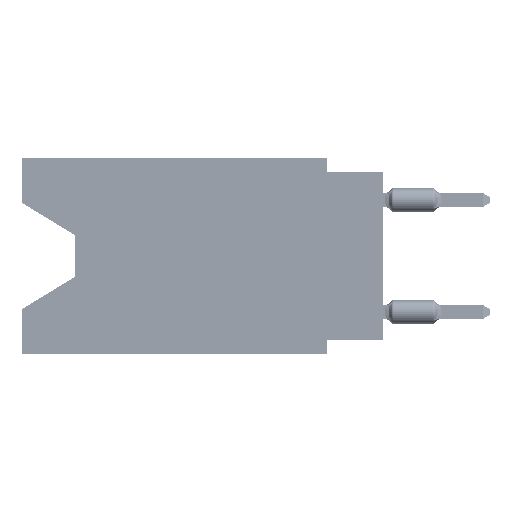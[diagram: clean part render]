
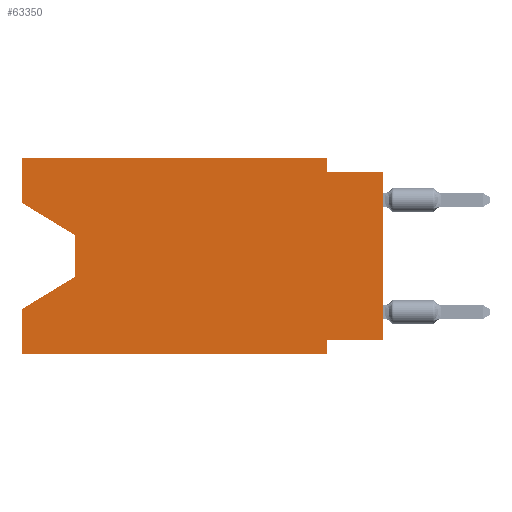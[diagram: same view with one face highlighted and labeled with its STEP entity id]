
A CAD part, left-side view. The second image highlights one B-rep face of the part: STEP entity #63350.
In plain terms, the highlighted planar face has unit normal (-1, 0, 0).
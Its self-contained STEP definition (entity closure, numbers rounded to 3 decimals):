
#516 = CARTESIAN_POINT ( 'NONE',  ( 0., 16.383, -8.89 ) ) ;
#523 = VERTEX_POINT ( 'NONE', #42212 ) ;
#1295 = ORIENTED_EDGE ( 'NONE', *, *, #9275, .T. ) ;
#1318 = CARTESIAN_POINT ( 'NONE',  ( 0., 16.383, 0. ) ) ;
#1437 = CARTESIAN_POINT ( 'NONE',  ( 0., 2.54, -0.635 ) ) ;
#3641 = CARTESIAN_POINT ( 'NONE',  ( 0., 16.383, -8.89 ) ) ;
#4313 = EDGE_LOOP ( 'NONE', ( #29457, #71817, #26919, #73479, #1295, #72727, #35749, #52453, #12389, #7463, #73319, #43682 ) ) ;
#5982 = EDGE_CURVE ( 'NONE', #16582, #79800, #67803, .T. ) ;
#7463 = ORIENTED_EDGE ( 'NONE', *, *, #47784, .F. ) ;
#7581 = VERTEX_POINT ( 'NONE', #72107 ) ;
#7831 = CARTESIAN_POINT ( 'NONE',  ( 0., 2.54, -8.89 ) ) ;
#9275 = EDGE_CURVE ( 'NONE', #50242, #82843, #55968, .T. ) ;
#9385 = CARTESIAN_POINT ( 'NONE',  ( 0., 16.383, 0. ) ) ;
#10523 = VECTOR ( 'NONE', #65945, 1000. ) ;
#11634 = VECTOR ( 'NONE', #74355, 1000. ) ;
#11672 = VERTEX_POINT ( 'NONE', #40028 ) ;
#12389 = ORIENTED_EDGE ( 'NONE', *, *, #19024, .F. ) ;
#14212 = DIRECTION ( 'NONE',  ( 0., 1., 0. ) ) ;
#16483 = VERTEX_POINT ( 'NONE', #26342 ) ;
#16582 = VERTEX_POINT ( 'NONE', #68584 ) ;
#18883 = DIRECTION ( 'NONE',  ( 0., 0., -1. ) ) ;
#19024 = EDGE_CURVE ( 'NONE', #61422, #16483, #24366, .T. ) ;
#19853 = EDGE_CURVE ( 'NONE', #7581, #58086, #46679, .T. ) ;
#20023 = DIRECTION ( 'NONE',  ( 1., 0., 0. ) ) ;
#21522 = VECTOR ( 'NONE', #34425, 1000. ) ;
#21980 = DIRECTION ( 'NONE',  ( 0., 0., 1. ) ) ;
#22402 = CARTESIAN_POINT ( 'NONE',  ( 0., 16.383, 0. ) ) ;
#24366 = LINE ( 'NONE', #50952, #11634 ) ;
#25097 = LINE ( 'NONE', #50391, #69013 ) ;
#25262 = FACE_OUTER_BOUND ( 'NONE', #4313, .T. ) ;
#26206 = CARTESIAN_POINT ( 'NONE',  ( 0., 13.97, -3.505 ) ) ;
#26342 = CARTESIAN_POINT ( 'NONE',  ( 0., 0., -0.635 ) ) ;
#26910 = EDGE_CURVE ( 'NONE', #79800, #82843, #40957, .T. ) ;
#26919 = ORIENTED_EDGE ( 'NONE', *, *, #42060, .T. ) ;
#27352 = LINE ( 'NONE', #47828, #77797 ) ;
#28202 = DIRECTION ( 'NONE',  ( 0., 0., 1. ) ) ;
#28610 = EDGE_CURVE ( 'NONE', #43066, #11672, #44593, .T. ) ;
#29457 = ORIENTED_EDGE ( 'NONE', *, *, #48262, .T. ) ;
#33030 = EDGE_CURVE ( 'NONE', #33920, #7581, #35910, .T. ) ;
#33920 = VERTEX_POINT ( 'NONE', #84054 ) ;
#34425 = DIRECTION ( 'NONE',  ( 0., 0., -1. ) ) ;
#34693 = CARTESIAN_POINT ( 'NONE',  ( 0., 2.54, -8.255 ) ) ;
#35749 = ORIENTED_EDGE ( 'NONE', *, *, #5982, .F. ) ;
#35910 = LINE ( 'NONE', #22402, #81858 ) ;
#37272 = LINE ( 'NONE', #9385, #57792 ) ;
#39633 = CARTESIAN_POINT ( 'NONE',  ( 0., 2.54, -8.89 ) ) ;
#40028 = CARTESIAN_POINT ( 'NONE',  ( 0., 13.97, -5.385 ) ) ;
#40957 = LINE ( 'NONE', #7831, #21522 ) ;
#41112 = VECTOR ( 'NONE', #14212, 1000. ) ;
#42060 = EDGE_CURVE ( 'NONE', #11672, #523, #49560, .T. ) ;
#42212 = CARTESIAN_POINT ( 'NONE',  ( 0., 16.383, -6.852 ) ) ;
#43066 = VERTEX_POINT ( 'NONE', #26206 ) ;
#43682 = ORIENTED_EDGE ( 'NONE', *, *, #33030, .F. ) ;
#44593 = LINE ( 'NONE', #78188, #74592 ) ;
#45731 = PLANE ( 'NONE',  #71780 ) ;
#46468 = CARTESIAN_POINT ( 'NONE',  ( 0., 0., -8.255 ) ) ;
#46679 = LINE ( 'NONE', #1318, #68872 ) ;
#47784 = EDGE_CURVE ( 'NONE', #58086, #61422, #25097, .T. ) ;
#47828 = CARTESIAN_POINT ( 'NONE',  ( 0., 0., 0. ) ) ;
#48262 = EDGE_CURVE ( 'NONE', #33920, #43066, #58981, .T. ) ;
#49006 = DIRECTION ( 'NONE',  ( 0., -1., 0. ) ) ;
#49560 = LINE ( 'NONE', #68757, #65703 ) ;
#50198 = CARTESIAN_POINT ( 'NONE',  ( 0., 2.54, 0. ) ) ;
#50242 = VERTEX_POINT ( 'NONE', #516 ) ;
#50391 = CARTESIAN_POINT ( 'NONE',  ( 0., 2.54, 0. ) ) ;
#50775 = DIRECTION ( 'NONE',  ( 0., 0., 1. ) ) ;
#50952 = CARTESIAN_POINT ( 'NONE',  ( 0., 0., -0.635 ) ) ;
#52453 = ORIENTED_EDGE ( 'NONE', *, *, #68764, .T. ) ;
#53579 = DIRECTION ( 'NONE',  ( 0., 0., -1. ) ) ;
#55968 = LINE ( 'NONE', #3641, #75243 ) ;
#57792 = VECTOR ( 'NONE', #50775, 1000. ) ;
#58086 = VERTEX_POINT ( 'NONE', #50198 ) ;
#58981 = LINE ( 'NONE', #73802, #10523 ) ;
#60538 = EDGE_CURVE ( 'NONE', #50242, #523, #37272, .T. ) ;
#61422 = VERTEX_POINT ( 'NONE', #1437 ) ;
#63350 = ADVANCED_FACE ( 'NONE', ( #25262 ), #45731, .F. ) ;
#65703 = VECTOR ( 'NONE', #75312, 1000. ) ;
#65945 = DIRECTION ( 'NONE',  ( 0., -0.855, -0.519 ) ) ;
#67803 = LINE ( 'NONE', #46468, #41112 ) ;
#68584 = CARTESIAN_POINT ( 'NONE',  ( 0., 0., -8.255 ) ) ;
#68757 = CARTESIAN_POINT ( 'NONE',  ( 0., 13.97, -5.385 ) ) ;
#68764 = EDGE_CURVE ( 'NONE', #16582, #16483, #27352, .T. ) ;
#68872 = VECTOR ( 'NONE', #80264, 1000. ) ;
#69013 = VECTOR ( 'NONE', #73044, 1000. ) ;
#71780 = AXIS2_PLACEMENT_3D ( 'NONE', #72331, #20023, #53579 ) ;
#71817 = ORIENTED_EDGE ( 'NONE', *, *, #28610, .T. ) ;
#72107 = CARTESIAN_POINT ( 'NONE',  ( 0., 16.383, 0. ) ) ;
#72331 = CARTESIAN_POINT ( 'NONE',  ( 0., 16.383, 0. ) ) ;
#72727 = ORIENTED_EDGE ( 'NONE', *, *, #26910, .F. ) ;
#73044 = DIRECTION ( 'NONE',  ( 0., 0., -1. ) ) ;
#73319 = ORIENTED_EDGE ( 'NONE', *, *, #19853, .F. ) ;
#73479 = ORIENTED_EDGE ( 'NONE', *, *, #60538, .F. ) ;
#73802 = CARTESIAN_POINT ( 'NONE',  ( 0., 16.383, -2.038 ) ) ;
#74355 = DIRECTION ( 'NONE',  ( 0., -1., 0. ) ) ;
#74592 = VECTOR ( 'NONE', #18883, 1000. ) ;
#75243 = VECTOR ( 'NONE', #49006, 1000. ) ;
#75312 = DIRECTION ( 'NONE',  ( 0., 0.855, -0.519 ) ) ;
#77797 = VECTOR ( 'NONE', #28202, 1000. ) ;
#78188 = CARTESIAN_POINT ( 'NONE',  ( 0., 13.97, -3.505 ) ) ;
#79800 = VERTEX_POINT ( 'NONE', #34693 ) ;
#80264 = DIRECTION ( 'NONE',  ( 0., -1., 0. ) ) ;
#81858 = VECTOR ( 'NONE', #21980, 1000. ) ;
#82843 = VERTEX_POINT ( 'NONE', #39633 ) ;
#84054 = CARTESIAN_POINT ( 'NONE',  ( 0., 16.383, -2.038 ) ) ;
